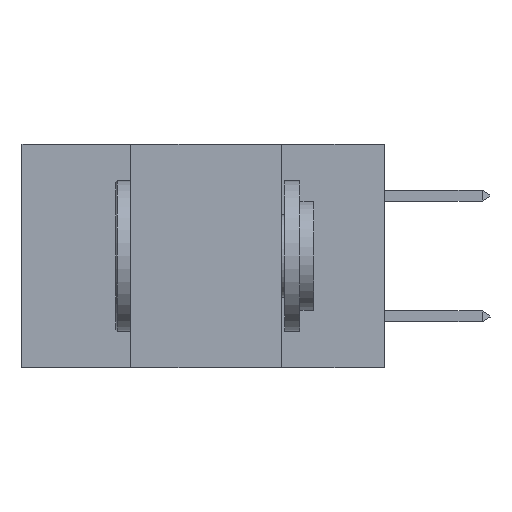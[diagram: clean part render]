
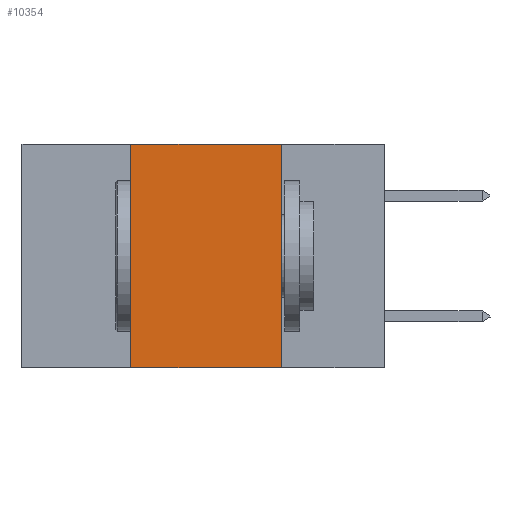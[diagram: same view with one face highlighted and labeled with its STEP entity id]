
A CAD part, left-side view. The second image highlights one B-rep face of the part: STEP entity #10354.
In plain terms, the highlighted planar face has unit normal (-1, 0, 0).
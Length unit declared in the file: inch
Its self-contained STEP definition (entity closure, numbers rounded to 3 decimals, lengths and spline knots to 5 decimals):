
#338 = DIRECTION ( 'NONE',  ( 0., -1., 0. ) ) ;
#1252 = EDGE_CURVE ( 'NONE', #14528, #22010, #7671, .T. ) ;
#1310 = CARTESIAN_POINT ( 'NONE',  ( 0., 0.17, -0.37 ) ) ;
#1611 = ORIENTED_EDGE ( 'NONE', *, *, #13298, .T. ) ;
#2747 = EDGE_CURVE ( 'NONE', #5145, #14528, #14956, .T. ) ;
#3216 = ORIENTED_EDGE ( 'NONE', *, *, #1252, .F. ) ;
#3918 = CARTESIAN_POINT ( 'NONE',  ( 0., 0.6, 0. ) ) ;
#4253 = VECTOR ( 'NONE', #338, 39.37008 ) ;
#4553 = DIRECTION ( 'NONE',  ( 0., -1., 0. ) ) ;
#4820 = EDGE_LOOP ( 'NONE', ( #18083, #3216, #5940, #1611 ) ) ;
#5145 = VERTEX_POINT ( 'NONE', #21586 ) ;
#5940 = ORIENTED_EDGE ( 'NONE', *, *, #2747, .F. ) ;
#6689 = CARTESIAN_POINT ( 'NONE',  ( 0., 0.6, 0. ) ) ;
#6836 = DIRECTION ( 'NONE',  ( 1., 0., 0. ) ) ;
#6926 = PLANE ( 'NONE',  #11471 ) ;
#7671 = LINE ( 'NONE', #3918, #4253 ) ;
#8918 = CARTESIAN_POINT ( 'NONE',  ( 0., 0.42, 0. ) ) ;
#9872 = CARTESIAN_POINT ( 'NONE',  ( 0., 0.17, 0. ) ) ;
#10018 = CARTESIAN_POINT ( 'NONE',  ( 0., 0.6, -0.37 ) ) ;
#10123 = VECTOR ( 'NONE', #17099, 39.37008 ) ;
#10354 = ADVANCED_FACE ( 'NONE', ( #23091 ), #6926, .F. ) ;
#10555 = DIRECTION ( 'NONE',  ( 0., 0., -1. ) ) ;
#10915 = CARTESIAN_POINT ( 'NONE',  ( 0., 0.42, 0. ) ) ;
#11471 = AXIS2_PLACEMENT_3D ( 'NONE', #6689, #6836, #10555 ) ;
#11821 = CARTESIAN_POINT ( 'NONE',  ( 0., 0.17, 0. ) ) ;
#12980 = VECTOR ( 'NONE', #4553, 39.37008 ) ;
#13298 = EDGE_CURVE ( 'NONE', #5145, #15030, #23179, .T. ) ;
#14528 = VERTEX_POINT ( 'NONE', #10915 ) ;
#14956 = LINE ( 'NONE', #8918, #20082 ) ;
#15030 = VERTEX_POINT ( 'NONE', #1310 ) ;
#17099 = DIRECTION ( 'NONE',  ( 0., 0., -1. ) ) ;
#17790 = LINE ( 'NONE', #9872, #10123 ) ;
#18083 = ORIENTED_EDGE ( 'NONE', *, *, #19680, .F. ) ;
#19680 = EDGE_CURVE ( 'NONE', #22010, #15030, #17790, .T. ) ;
#19882 = DIRECTION ( 'NONE',  ( 0., 0., 1. ) ) ;
#20082 = VECTOR ( 'NONE', #19882, 39.37008 ) ;
#21586 = CARTESIAN_POINT ( 'NONE',  ( 0., 0.42, -0.37 ) ) ;
#22010 = VERTEX_POINT ( 'NONE', #11821 ) ;
#23091 = FACE_OUTER_BOUND ( 'NONE', #4820, .T. ) ;
#23179 = LINE ( 'NONE', #10018, #12980 ) ;
